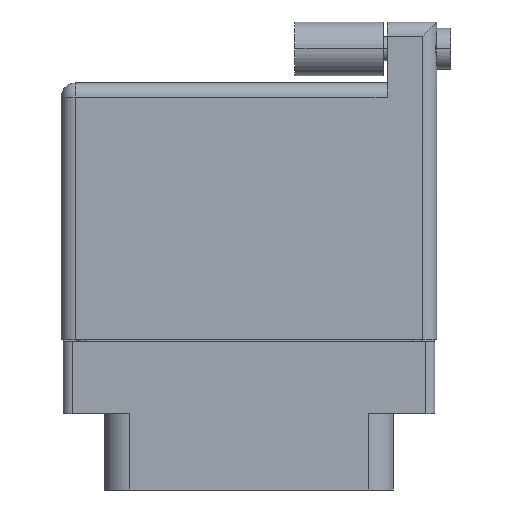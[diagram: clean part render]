
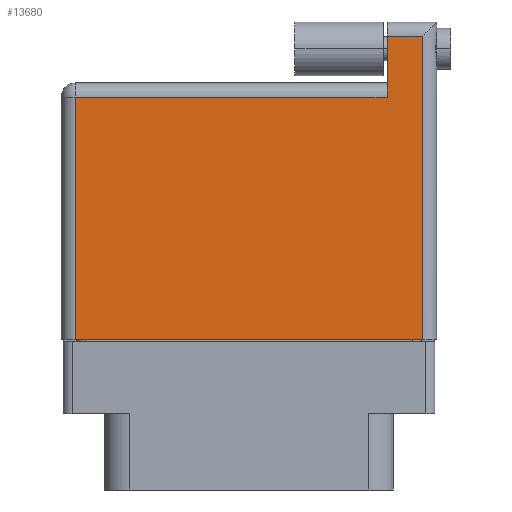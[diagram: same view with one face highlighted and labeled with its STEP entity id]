
A CAD part, front view. The second image highlights one B-rep face of the part: STEP entity #13680.
In plain terms, the highlighted face is planar.
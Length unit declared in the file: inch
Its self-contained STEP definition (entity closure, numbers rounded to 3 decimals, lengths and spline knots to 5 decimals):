
#252 = DIRECTION ( 'NONE',  ( 0., -1., 0. ) ) ;
#874 = EDGE_CURVE ( 'NONE', #23530, #4674, #4543, .T. ) ;
#1241 = VECTOR ( 'NONE', #9477, 39.37008 ) ;
#2114 = CARTESIAN_POINT ( 'NONE',  ( 0.4875, 1.02, 0.3575 ) ) ;
#2720 = ORIENTED_EDGE ( 'NONE', *, *, #12839, .T. ) ;
#2964 = LINE ( 'NONE', #18557, #14854 ) ;
#4413 = CARTESIAN_POINT ( 'NONE',  ( -0.6625, -0.1, 0.3575 ) ) ;
#4421 = CARTESIAN_POINT ( 'NONE',  ( 0.6125, 0.97, 0.3575 ) ) ;
#4543 = LINE ( 'NONE', #4413, #6491 ) ;
#4674 = VERTEX_POINT ( 'NONE', #8555 ) ;
#4808 = DIRECTION ( 'NONE',  ( -1., 0., 0. ) ) ;
#4823 = ORIENTED_EDGE ( 'NONE', *, *, #10237, .T. ) ;
#6135 = CARTESIAN_POINT ( 'NONE',  ( -0.6625, 0.806, 0.3575 ) ) ;
#6245 = CARTESIAN_POINT ( 'NONE',  ( -0.6125, -0.1, 0.3575 ) ) ;
#6491 = VECTOR ( 'NONE', #18674, 39.37008 ) ;
#7656 = EDGE_LOOP ( 'NONE', ( #7905, #19157, #4823, #2720, #10900, #9463 ) ) ;
#7905 = ORIENTED_EDGE ( 'NONE', *, *, #874, .T. ) ;
#7977 = CARTESIAN_POINT ( 'NONE',  ( -0.6125, -0.1, 0.3575 ) ) ;
#8481 = CARTESIAN_POINT ( 'NONE',  ( 0.4875, 0.756, 0.3575 ) ) ;
#8555 = CARTESIAN_POINT ( 'NONE',  ( 0.6125, -0.1, 0.3575 ) ) ;
#9233 = VECTOR ( 'NONE', #252, 39.37008 ) ;
#9463 = ORIENTED_EDGE ( 'NONE', *, *, #14078, .T. ) ;
#9477 = DIRECTION ( 'NONE',  ( 0., 1., 0. ) ) ;
#9762 = AXIS2_PLACEMENT_3D ( 'NONE', #6135, #14454, #10095 ) ;
#10095 = DIRECTION ( 'NONE',  ( -1., 0., 0. ) ) ;
#10237 = EDGE_CURVE ( 'NONE', #20905, #22191, #2964, .T. ) ;
#10900 = ORIENTED_EDGE ( 'NONE', *, *, #19854, .T. ) ;
#11002 = DIRECTION ( 'NONE',  ( -1., 0., 0. ) ) ;
#11591 = CARTESIAN_POINT ( 'NONE',  ( 0.6125, 1.02, 0.3575 ) ) ;
#11655 = VERTEX_POINT ( 'NONE', #21241 ) ;
#12839 = EDGE_CURVE ( 'NONE', #22191, #22768, #20204, .T. ) ;
#13680 = ADVANCED_FACE ( 'NONE', ( #14324 ), #14600, .F. ) ;
#14078 = EDGE_CURVE ( 'NONE', #11655, #23530, #24483, .T. ) ;
#14324 = FACE_OUTER_BOUND ( 'NONE', #7656, .T. ) ;
#14454 = DIRECTION ( 'NONE',  ( 0., 0., -1. ) ) ;
#14600 = PLANE ( 'NONE',  #9762 ) ;
#14832 = LINE ( 'NONE', #20917, #16718 ) ;
#14854 = VECTOR ( 'NONE', #11002, 39.37008 ) ;
#16718 = VECTOR ( 'NONE', #4808, 39.37008 ) ;
#18107 = EDGE_CURVE ( 'NONE', #4674, #20905, #25733, .T. ) ;
#18130 = DIRECTION ( 'NONE',  ( 0., -1., 0. ) ) ;
#18557 = CARTESIAN_POINT ( 'NONE',  ( -0.6625, 0.97, 0.3575 ) ) ;
#18674 = DIRECTION ( 'NONE',  ( 1., 0., 0. ) ) ;
#19157 = ORIENTED_EDGE ( 'NONE', *, *, #18107, .T. ) ;
#19854 = EDGE_CURVE ( 'NONE', #22768, #11655, #14832, .T. ) ;
#20204 = LINE ( 'NONE', #2114, #9233 ) ;
#20801 = VECTOR ( 'NONE', #18130, 39.37008 ) ;
#20905 = VERTEX_POINT ( 'NONE', #4421 ) ;
#20917 = CARTESIAN_POINT ( 'NONE',  ( -0.6625, 0.756, 0.3575 ) ) ;
#21241 = CARTESIAN_POINT ( 'NONE',  ( -0.6125, 0.756, 0.3575 ) ) ;
#22011 = CARTESIAN_POINT ( 'NONE',  ( 0.4875, 0.97, 0.3575 ) ) ;
#22191 = VERTEX_POINT ( 'NONE', #22011 ) ;
#22768 = VERTEX_POINT ( 'NONE', #8481 ) ;
#23530 = VERTEX_POINT ( 'NONE', #7977 ) ;
#24483 = LINE ( 'NONE', #6245, #20801 ) ;
#25733 = LINE ( 'NONE', #11591, #1241 ) ;
